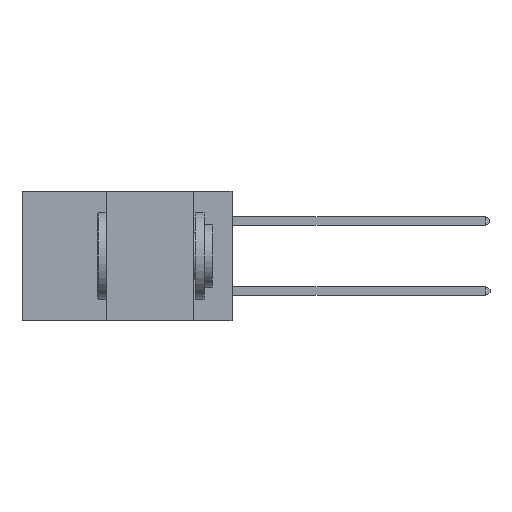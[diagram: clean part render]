
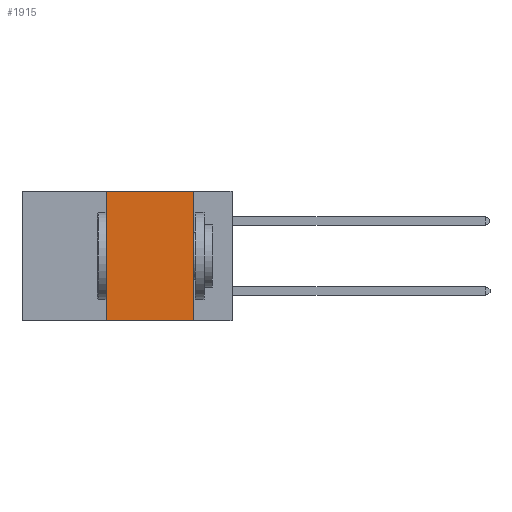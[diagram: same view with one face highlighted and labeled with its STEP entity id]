
A CAD part, left-side view. The second image highlights one B-rep face of the part: STEP entity #1915.
In plain terms, the highlighted planar face has unit normal (-1, 0, 0).
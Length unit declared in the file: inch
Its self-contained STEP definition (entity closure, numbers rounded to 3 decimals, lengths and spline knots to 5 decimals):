
#289 = ORIENTED_EDGE ( 'NONE', *, *, #4314, .F. ) ;
#986 = DIRECTION ( 'NONE',  ( 0., 0., -1. ) ) ;
#996 = EDGE_CURVE ( 'NONE', #14355, #1019, #10115, .T. ) ;
#1019 = VERTEX_POINT ( 'NONE', #9775 ) ;
#1472 = DIRECTION ( 'NONE',  ( 1., 0., 0. ) ) ;
#1915 = ADVANCED_FACE ( 'NONE', ( #13168 ), #4083, .F. ) ;
#3270 = CARTESIAN_POINT ( 'NONE',  ( 0., 0.6, 0. ) ) ;
#4083 = PLANE ( 'NONE',  #15299 ) ;
#4314 = EDGE_CURVE ( 'NONE', #14355, #14390, #17491, .T. ) ;
#5347 = VECTOR ( 'NONE', #7526, 39.37008 ) ;
#5779 = EDGE_CURVE ( 'NONE', #10626, #1019, #10143, .T. ) ;
#6454 = VECTOR ( 'NONE', #10215, 39.37008 ) ;
#6533 = CARTESIAN_POINT ( 'NONE',  ( 0., 0.11, 0. ) ) ;
#7526 = DIRECTION ( 'NONE',  ( 0., -1., 0. ) ) ;
#7535 = ORIENTED_EDGE ( 'NONE', *, *, #5779, .F. ) ;
#9528 = CARTESIAN_POINT ( 'NONE',  ( 0., 0.36, -0.37 ) ) ;
#9775 = CARTESIAN_POINT ( 'NONE',  ( 0., 0.11, -0.37 ) ) ;
#9945 = DIRECTION ( 'NONE',  ( 0., -1., 0. ) ) ;
#10115 = LINE ( 'NONE', #10126, #16820 ) ;
#10126 = CARTESIAN_POINT ( 'NONE',  ( 0., 0.6, -0.37 ) ) ;
#10143 = LINE ( 'NONE', #12369, #6454 ) ;
#10215 = DIRECTION ( 'NONE',  ( 0., 0., -1. ) ) ;
#10626 = VERTEX_POINT ( 'NONE', #6533 ) ;
#10951 = CARTESIAN_POINT ( 'NONE',  ( 0., 0.36, 0. ) ) ;
#12321 = LINE ( 'NONE', #14464, #5347 ) ;
#12369 = CARTESIAN_POINT ( 'NONE',  ( 0., 0.11, 0. ) ) ;
#13168 = FACE_OUTER_BOUND ( 'NONE', #17289, .T. ) ;
#14195 = EDGE_CURVE ( 'NONE', #14390, #10626, #12321, .T. ) ;
#14355 = VERTEX_POINT ( 'NONE', #9528 ) ;
#14390 = VERTEX_POINT ( 'NONE', #10951 ) ;
#14464 = CARTESIAN_POINT ( 'NONE',  ( 0., 0.6, 0. ) ) ;
#14913 = ORIENTED_EDGE ( 'NONE', *, *, #14195, .F. ) ;
#15160 = DIRECTION ( 'NONE',  ( 0., 0., 1. ) ) ;
#15241 = CARTESIAN_POINT ( 'NONE',  ( 0., 0.36, 0. ) ) ;
#15299 = AXIS2_PLACEMENT_3D ( 'NONE', #3270, #1472, #986 ) ;
#15347 = ORIENTED_EDGE ( 'NONE', *, *, #996, .T. ) ;
#16820 = VECTOR ( 'NONE', #9945, 39.37008 ) ;
#17071 = VECTOR ( 'NONE', #15160, 39.37008 ) ;
#17289 = EDGE_LOOP ( 'NONE', ( #7535, #14913, #289, #15347 ) ) ;
#17491 = LINE ( 'NONE', #15241, #17071 ) ;
